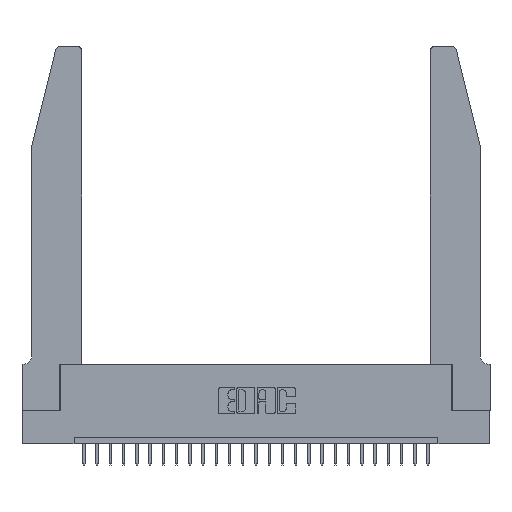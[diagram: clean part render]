
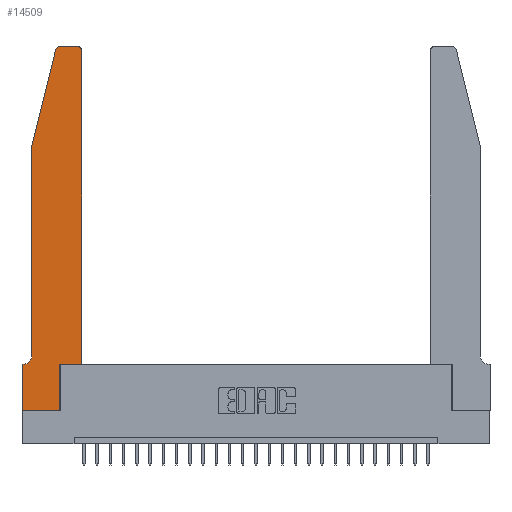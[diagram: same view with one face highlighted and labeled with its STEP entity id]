
A CAD part, top view. The second image highlights one B-rep face of the part: STEP entity #14509.
In plain terms, the highlighted planar face has unit normal (0, 0, 1).
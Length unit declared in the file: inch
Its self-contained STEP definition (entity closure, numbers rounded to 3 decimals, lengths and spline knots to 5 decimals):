
#4 = EDGE_LOOP ( 'NONE', ( #10157, #17005, #8761, #27064, #19989, #2370, #10184, #22158, #9108, #25962, #14074, #3998 ) ) ;
#109 = CARTESIAN_POINT ( 'NONE',  ( 0.4505, 2.72, 0.37 ) ) ;
#128 = VECTOR ( 'NONE', #15168, 39.37008 ) ;
#225 = DIRECTION ( 'NONE',  ( 0., -1., 0. ) ) ;
#385 = CIRCLE ( 'NONE', #24509, 0.07 ) ;
#445 = AXIS2_PLACEMENT_3D ( 'NONE', #15857, #19997, #7656 ) ;
#640 = CARTESIAN_POINT ( 'NONE',  ( 0.0755, 2., 0.37 ) ) ;
#735 = VECTOR ( 'NONE', #225, 39.37008 ) ;
#768 = CARTESIAN_POINT ( 'NONE',  ( 0.284, 2.75, 0.37 ) ) ;
#1365 = CARTESIAN_POINT ( 'NONE',  ( 0.0755, 0.42, 0.37 ) ) ;
#1405 = PLANE ( 'NONE',  #445 ) ;
#2305 = CARTESIAN_POINT ( 'NONE',  ( 0.284, 2.72, 0.37 ) ) ;
#2331 = EDGE_CURVE ( 'NONE', #7509, #19684, #25699, .T. ) ;
#2370 = ORIENTED_EDGE ( 'NONE', *, *, #19448, .T. ) ;
#2731 = CARTESIAN_POINT ( 'NONE',  ( 0.4505, 0.35, 0.37 ) ) ;
#2876 = CARTESIAN_POINT ( 'NONE',  ( 0.0755, 0.35, 0.37 ) ) ;
#3214 = CARTESIAN_POINT ( 'NONE',  ( 0., 0., 0.37 ) ) ;
#3998 = ORIENTED_EDGE ( 'NONE', *, *, #2331, .T. ) ;
#4091 = EDGE_CURVE ( 'NONE', #24277, #9132, #11526, .T. ) ;
#4400 = DIRECTION ( 'NONE',  ( 1., 0., 0. ) ) ;
#4717 = FACE_OUTER_BOUND ( 'NONE', #4, .T. ) ;
#4799 = CARTESIAN_POINT ( 'NONE',  ( 0.0055, 0.35, 0.37 ) ) ;
#4869 = LINE ( 'NONE', #640, #11439 ) ;
#5622 = VECTOR ( 'NONE', #17348, 39.37008 ) ;
#5667 = CARTESIAN_POINT ( 'NONE',  ( 0., 0.35, 0.37 ) ) ;
#6523 = EDGE_CURVE ( 'NONE', #6878, #7568, #16625, .T. ) ;
#6620 = DIRECTION ( 'NONE',  ( 0., 0., 1. ) ) ;
#6878 = VERTEX_POINT ( 'NONE', #3214 ) ;
#6901 = CARTESIAN_POINT ( 'NONE',  ( 0.2865, 0.35, 0.37 ) ) ;
#7048 = EDGE_CURVE ( 'NONE', #19684, #18796, #26417, .T. ) ;
#7259 = VERTEX_POINT ( 'NONE', #15310 ) ;
#7509 = VERTEX_POINT ( 'NONE', #109 ) ;
#7568 = VERTEX_POINT ( 'NONE', #12884 ) ;
#7656 = DIRECTION ( 'NONE',  ( 1., 0., 0. ) ) ;
#8107 = VECTOR ( 'NONE', #24991, 39.37008 ) ;
#8761 = ORIENTED_EDGE ( 'NONE', *, *, #11051, .T. ) ;
#8938 = CARTESIAN_POINT ( 'NONE',  ( 0.2605, 2.75, 0.37 ) ) ;
#9108 = ORIENTED_EDGE ( 'NONE', *, *, #17346, .T. ) ;
#9132 = VERTEX_POINT ( 'NONE', #2731 ) ;
#10018 = LINE ( 'NONE', #16275, #20806 ) ;
#10157 = ORIENTED_EDGE ( 'NONE', *, *, #7048, .T. ) ;
#10184 = ORIENTED_EDGE ( 'NONE', *, *, #24890, .T. ) ;
#10469 = AXIS2_PLACEMENT_3D ( 'NONE', #23651, #11123, #25762 ) ;
#11051 = EDGE_CURVE ( 'NONE', #23818, #7259, #4869, .T. ) ;
#11123 = DIRECTION ( 'NONE',  ( 0., 0., 1. ) ) ;
#11439 = VECTOR ( 'NONE', #15548, 39.37008 ) ;
#11526 = LINE ( 'NONE', #23163, #24296 ) ;
#11647 = VERTEX_POINT ( 'NONE', #4799 ) ;
#11852 = CARTESIAN_POINT ( 'NONE',  ( 0.4205, 2.75, 0.37 ) ) ;
#12877 = LINE ( 'NONE', #21200, #735 ) ;
#12884 = CARTESIAN_POINT ( 'NONE',  ( 0.2865, 0., 0.37 ) ) ;
#14049 = DIRECTION ( 'NONE',  ( -1., 0., 0. ) ) ;
#14074 = ORIENTED_EDGE ( 'NONE', *, *, #15539, .T. ) ;
#14509 = ADVANCED_FACE ( 'NONE', ( #4717 ), #1405, .T. ) ;
#14694 = EDGE_CURVE ( 'NONE', #20534, #11647, #385, .T. ) ;
#14750 = EDGE_CURVE ( 'NONE', #7259, #20534, #12877, .T. ) ;
#15168 = DIRECTION ( 'NONE',  ( 0., 1., 0. ) ) ;
#15222 = CARTESIAN_POINT ( 'NONE',  ( 0.4505, 0.35, 0.37 ) ) ;
#15310 = CARTESIAN_POINT ( 'NONE',  ( 0.0755, 2., 0.37 ) ) ;
#15539 = EDGE_CURVE ( 'NONE', #9132, #7509, #22325, .T. ) ;
#15548 = DIRECTION ( 'NONE',  ( -0.239, -0.971, 0. ) ) ;
#15857 = CARTESIAN_POINT ( 'NONE',  ( 0., 0.35, 0.37 ) ) ;
#16275 = CARTESIAN_POINT ( 'NONE',  ( 0., 0., 0.37 ) ) ;
#16625 = LINE ( 'NONE', #22789, #8107 ) ;
#16779 = CIRCLE ( 'NONE', #20547, 0.03 ) ;
#17005 = ORIENTED_EDGE ( 'NONE', *, *, #20359, .T. ) ;
#17346 = EDGE_CURVE ( 'NONE', #7568, #24277, #21428, .T. ) ;
#17348 = DIRECTION ( 'NONE',  ( 0., 1., 0. ) ) ;
#18347 = VERTEX_POINT ( 'NONE', #5667 ) ;
#18796 = VERTEX_POINT ( 'NONE', #768 ) ;
#18880 = VECTOR ( 'NONE', #14049, 39.37008 ) ;
#19002 = DIRECTION ( 'NONE',  ( 0., 0., -1. ) ) ;
#19448 = EDGE_CURVE ( 'NONE', #11647, #18347, #21348, .T. ) ;
#19684 = VERTEX_POINT ( 'NONE', #11852 ) ;
#19989 = ORIENTED_EDGE ( 'NONE', *, *, #14694, .T. ) ;
#19997 = DIRECTION ( 'NONE',  ( 0., 0., 1. ) ) ;
#20359 = EDGE_CURVE ( 'NONE', #18796, #23818, #16779, .T. ) ;
#20440 = CARTESIAN_POINT ( 'NONE',  ( 0.2865, 0.35, 0.37 ) ) ;
#20534 = VERTEX_POINT ( 'NONE', #1365 ) ;
#20547 = AXIS2_PLACEMENT_3D ( 'NONE', #2305, #6620, #23464 ) ;
#20806 = VECTOR ( 'NONE', #24927, 39.37008 ) ;
#21149 = DIRECTION ( 'NONE',  ( -1., 0., 0. ) ) ;
#21200 = CARTESIAN_POINT ( 'NONE',  ( 0.0755, 2., 0.37 ) ) ;
#21348 = LINE ( 'NONE', #2876, #26313 ) ;
#21428 = LINE ( 'NONE', #6901, #128 ) ;
#21706 = DIRECTION ( 'NONE',  ( -1., 0., 0. ) ) ;
#22158 = ORIENTED_EDGE ( 'NONE', *, *, #6523, .T. ) ;
#22325 = LINE ( 'NONE', #15222, #5622 ) ;
#22789 = CARTESIAN_POINT ( 'NONE',  ( 0., 0., 0.37 ) ) ;
#23163 = CARTESIAN_POINT ( 'NONE',  ( 0.4505, 0.35, 0.37 ) ) ;
#23464 = DIRECTION ( 'NONE',  ( 1., 0., 0. ) ) ;
#23520 = CARTESIAN_POINT ( 'NONE',  ( 0.25487, 2.72718, 0.37 ) ) ;
#23651 = CARTESIAN_POINT ( 'NONE',  ( 0.4205, 2.72, 0.37 ) ) ;
#23818 = VERTEX_POINT ( 'NONE', #23520 ) ;
#24277 = VERTEX_POINT ( 'NONE', #20440 ) ;
#24296 = VECTOR ( 'NONE', #4400, 39.37008 ) ;
#24509 = AXIS2_PLACEMENT_3D ( 'NONE', #27042, #19002, #21149 ) ;
#24890 = EDGE_CURVE ( 'NONE', #18347, #6878, #10018, .T. ) ;
#24927 = DIRECTION ( 'NONE',  ( 0., -1., 0. ) ) ;
#24991 = DIRECTION ( 'NONE',  ( 1., 0., 0. ) ) ;
#25699 = CIRCLE ( 'NONE', #10469, 0.03 ) ;
#25762 = DIRECTION ( 'NONE',  ( 1., 0., 0. ) ) ;
#25962 = ORIENTED_EDGE ( 'NONE', *, *, #4091, .T. ) ;
#26313 = VECTOR ( 'NONE', #21706, 39.37008 ) ;
#26417 = LINE ( 'NONE', #8938, #18880 ) ;
#27042 = CARTESIAN_POINT ( 'NONE',  ( 0.0055, 0.42, 0.37 ) ) ;
#27064 = ORIENTED_EDGE ( 'NONE', *, *, #14750, .T. ) ;
